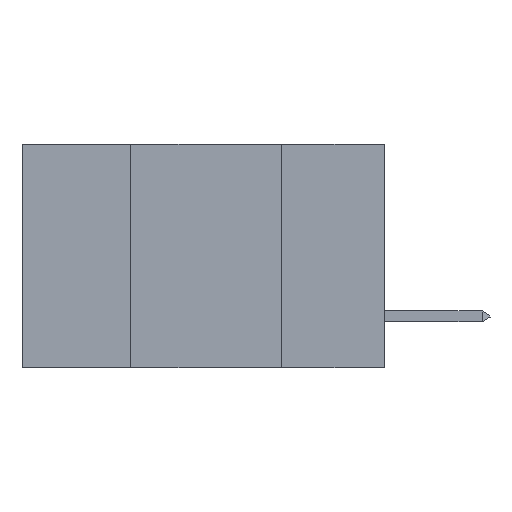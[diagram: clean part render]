
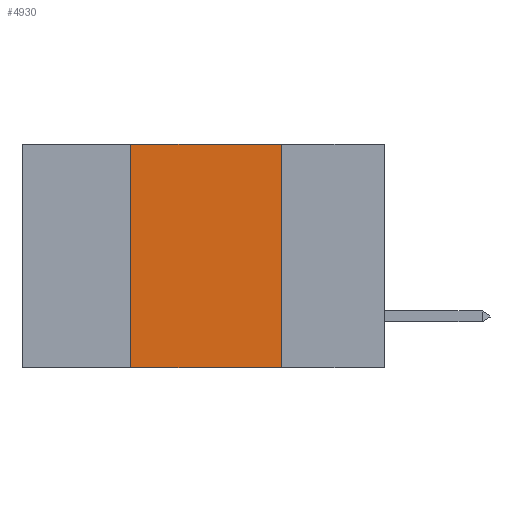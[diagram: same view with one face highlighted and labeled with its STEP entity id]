
A CAD part, left-side view. The second image highlights one B-rep face of the part: STEP entity #4930.
In plain terms, the highlighted planar face has unit normal (-1, 0, 0).
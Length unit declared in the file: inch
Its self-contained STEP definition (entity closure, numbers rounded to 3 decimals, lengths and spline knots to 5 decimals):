
#69 = EDGE_CURVE ( 'NONE', #4879, #10095, #3542, .T. ) ;
#90 = VERTEX_POINT ( 'NONE', #2202 ) ;
#531 = EDGE_CURVE ( 'NONE', #90, #10095, #9639, .T. ) ;
#625 = LINE ( 'NONE', #9170, #12369 ) ;
#1509 = CARTESIAN_POINT ( 'NONE',  ( 0., 0.6, -0.37 ) ) ;
#1578 = DIRECTION ( 'NONE',  ( 0., 0., -1. ) ) ;
#1823 = CARTESIAN_POINT ( 'NONE',  ( 0., 0.6, 0. ) ) ;
#1857 = ORIENTED_EDGE ( 'NONE', *, *, #1976, .F. ) ;
#1976 = EDGE_CURVE ( 'NONE', #4879, #7776, #625, .T. ) ;
#2202 = CARTESIAN_POINT ( 'NONE',  ( 0., 0.17, 0. ) ) ;
#2266 = VECTOR ( 'NONE', #1578, 39.37008 ) ;
#2975 = DIRECTION ( 'NONE',  ( 1., 0., 0. ) ) ;
#3542 = LINE ( 'NONE', #1509, #4763 ) ;
#3568 = ORIENTED_EDGE ( 'NONE', *, *, #531, .F. ) ;
#4763 = VECTOR ( 'NONE', #12825, 39.37008 ) ;
#4879 = VERTEX_POINT ( 'NONE', #11043 ) ;
#4930 = ADVANCED_FACE ( 'NONE', ( #6338 ), #8551, .F. ) ;
#4995 = CARTESIAN_POINT ( 'NONE',  ( 0., 0.42, 0. ) ) ;
#6338 = FACE_OUTER_BOUND ( 'NONE', #12833, .T. ) ;
#6551 = DIRECTION ( 'NONE',  ( 0., -1., 0. ) ) ;
#6979 = DIRECTION ( 'NONE',  ( 0., 0., 1. ) ) ;
#7776 = VERTEX_POINT ( 'NONE', #4995 ) ;
#8163 = EDGE_CURVE ( 'NONE', #7776, #90, #11816, .T. ) ;
#8551 = PLANE ( 'NONE',  #12704 ) ;
#9170 = CARTESIAN_POINT ( 'NONE',  ( 0., 0.42, 0. ) ) ;
#9358 = CARTESIAN_POINT ( 'NONE',  ( 0., 0.17, -0.37 ) ) ;
#9639 = LINE ( 'NONE', #10125, #2266 ) ;
#10062 = ORIENTED_EDGE ( 'NONE', *, *, #8163, .F. ) ;
#10095 = VERTEX_POINT ( 'NONE', #9358 ) ;
#10125 = CARTESIAN_POINT ( 'NONE',  ( 0., 0.17, 0. ) ) ;
#10363 = ORIENTED_EDGE ( 'NONE', *, *, #69, .T. ) ;
#11043 = CARTESIAN_POINT ( 'NONE',  ( 0., 0.42, -0.37 ) ) ;
#11816 = LINE ( 'NONE', #13255, #14430 ) ;
#12369 = VECTOR ( 'NONE', #6979, 39.37008 ) ;
#12704 = AXIS2_PLACEMENT_3D ( 'NONE', #1823, #2975, #14163 ) ;
#12825 = DIRECTION ( 'NONE',  ( 0., -1., 0. ) ) ;
#12833 = EDGE_LOOP ( 'NONE', ( #3568, #10062, #1857, #10363 ) ) ;
#13255 = CARTESIAN_POINT ( 'NONE',  ( 0., 0.6, 0. ) ) ;
#14163 = DIRECTION ( 'NONE',  ( 0., 0., -1. ) ) ;
#14430 = VECTOR ( 'NONE', #6551, 39.37008 ) ;
